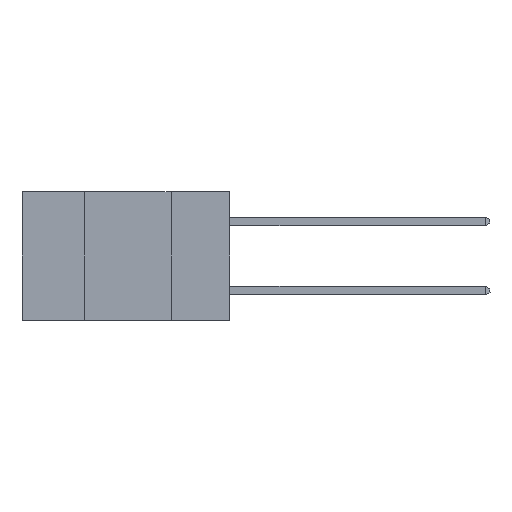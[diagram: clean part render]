
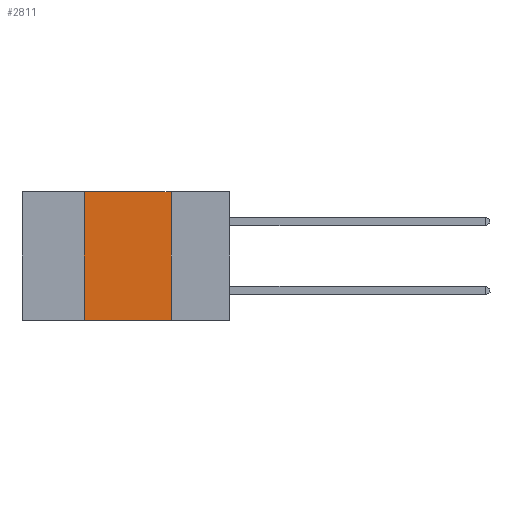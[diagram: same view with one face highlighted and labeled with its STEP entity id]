
A CAD part, left-side view. The second image highlights one B-rep face of the part: STEP entity #2811.
In plain terms, the highlighted planar face has unit normal (-1, 0, 0).
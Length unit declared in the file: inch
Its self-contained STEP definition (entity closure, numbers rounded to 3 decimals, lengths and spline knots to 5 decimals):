
#2327 = VERTEX_POINT ( 'NONE', #8310 ) ;
#2811 = ADVANCED_FACE ( 'NONE', ( #8079 ), #24123, .F. ) ;
#2913 = VERTEX_POINT ( 'NONE', #12097 ) ;
#3296 = DIRECTION ( 'NONE',  ( 0., 0., -1. ) ) ;
#3492 = CARTESIAN_POINT ( 'NONE',  ( 0., 0.17, 0. ) ) ;
#3806 = EDGE_LOOP ( 'NONE', ( #18754, #21092, #27279, #10346 ) ) ;
#6021 = EDGE_CURVE ( 'NONE', #2913, #20746, #20795, .T. ) ;
#6333 = VECTOR ( 'NONE', #18083, 39.37008 ) ;
#8079 = FACE_OUTER_BOUND ( 'NONE', #3806, .T. ) ;
#8310 = CARTESIAN_POINT ( 'NONE',  ( 0., 0.17, -0.37 ) ) ;
#9734 = CARTESIAN_POINT ( 'NONE',  ( 0., 0.6, -0.37 ) ) ;
#10091 = DIRECTION ( 'NONE',  ( 0., -1., 0. ) ) ;
#10346 = ORIENTED_EDGE ( 'NONE', *, *, #17118, .T. ) ;
#11221 = LINE ( 'NONE', #16403, #21796 ) ;
#12097 = CARTESIAN_POINT ( 'NONE',  ( 0., 0.42, -0.37 ) ) ;
#12598 = EDGE_CURVE ( 'NONE', #20746, #27151, #11221, .T. ) ;
#12608 = LINE ( 'NONE', #9734, #6333 ) ;
#13156 = VECTOR ( 'NONE', #20254, 39.37008 ) ;
#16100 = VECTOR ( 'NONE', #19350, 39.37008 ) ;
#16233 = CARTESIAN_POINT ( 'NONE',  ( 0., 0.17, 0. ) ) ;
#16403 = CARTESIAN_POINT ( 'NONE',  ( 0., 0.6, 0. ) ) ;
#17118 = EDGE_CURVE ( 'NONE', #2913, #2327, #12608, .T. ) ;
#17433 = LINE ( 'NONE', #16233, #16100 ) ;
#18083 = DIRECTION ( 'NONE',  ( 0., -1., 0. ) ) ;
#18705 = CARTESIAN_POINT ( 'NONE',  ( 0., 0.42, 0. ) ) ;
#18754 = ORIENTED_EDGE ( 'NONE', *, *, #26415, .F. ) ;
#19350 = DIRECTION ( 'NONE',  ( 0., 0., -1. ) ) ;
#20073 = CARTESIAN_POINT ( 'NONE',  ( 0., 0.6, 0. ) ) ;
#20254 = DIRECTION ( 'NONE',  ( 0., 0., 1. ) ) ;
#20746 = VERTEX_POINT ( 'NONE', #18705 ) ;
#20795 = LINE ( 'NONE', #22612, #13156 ) ;
#21092 = ORIENTED_EDGE ( 'NONE', *, *, #12598, .F. ) ;
#21796 = VECTOR ( 'NONE', #10091, 39.37008 ) ;
#22612 = CARTESIAN_POINT ( 'NONE',  ( 0., 0.42, 0. ) ) ;
#24123 = PLANE ( 'NONE',  #25655 ) ;
#25655 = AXIS2_PLACEMENT_3D ( 'NONE', #20073, #26465, #3296 ) ;
#26415 = EDGE_CURVE ( 'NONE', #27151, #2327, #17433, .T. ) ;
#26465 = DIRECTION ( 'NONE',  ( 1., 0., 0. ) ) ;
#27151 = VERTEX_POINT ( 'NONE', #3492 ) ;
#27279 = ORIENTED_EDGE ( 'NONE', *, *, #6021, .F. ) ;
